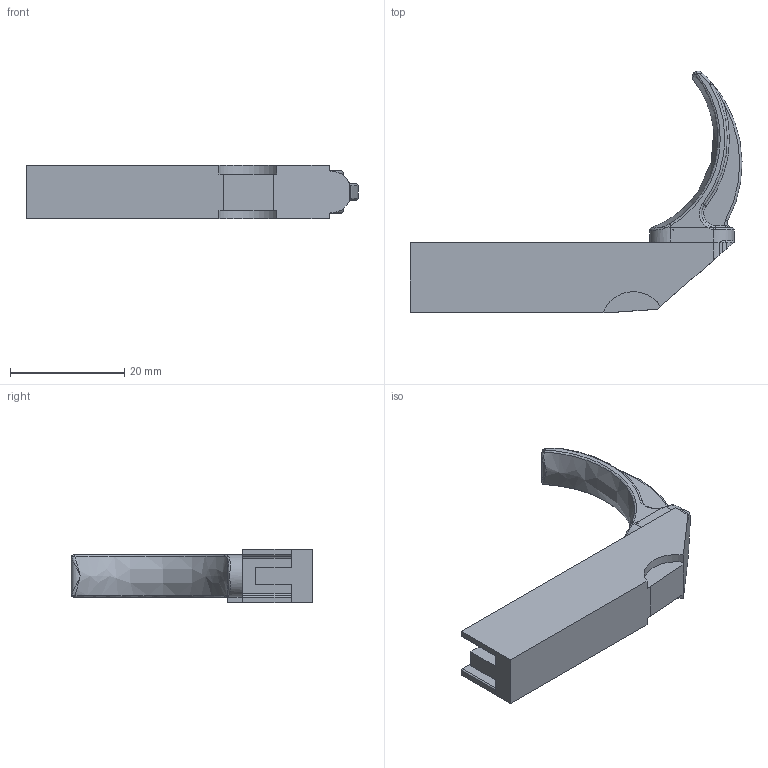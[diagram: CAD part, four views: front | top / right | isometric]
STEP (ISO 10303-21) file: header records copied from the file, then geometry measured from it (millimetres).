
FILE_DESCRIPTION(/* description */ (''),/* implementation_level */ '2;1');
FILE_NAME(/* name */ 'EpoxyTrigger-Curved.step',/* time_stamp */ '2020-10-31T22:01:08-04:00',/* author */ (''),/* organization */ (''),/* preprocessor_version */ 'ST-DEVELOPER v18.1',/* originating_system */ 'Autodesk Translation Framework v9.3.0.1241',/* authorisation */ '');
FILE_SCHEMA (('AUTOMOTIVE_DESIGN { 1 0 10303 214 3 1 1 }'));
Length unit declared in the file: millimetre
Products named in the file (1): Trigger
Bounding box: 58.06 x 42.25 x 9.37 mm (x, y, z)
Volume: 6150 mm3; surface area: 3570.1 mm2
Topology: 2 solids, 2 shells, 127 faces, 335 edges, 205 vertices
Faces by surface type: bspline 40, plane 34, cylinder 29, torus 22, sphere 2
Entity records: 13489 total; most frequent: CARTESIAN_POINT 10594, ORIENTED_EDGE 656, DIRECTION 525, EDGE_CURVE 328, VERTEX_POINT 205, AXIS2_PLACEMENT_3D 202, FACE_OUTER_BOUND 127, EDGE_LOOP 127
